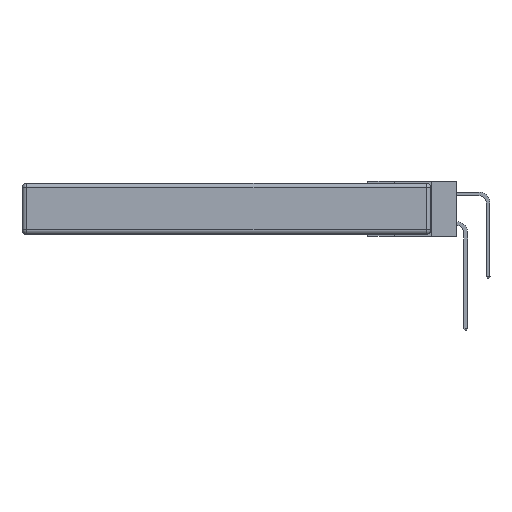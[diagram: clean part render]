
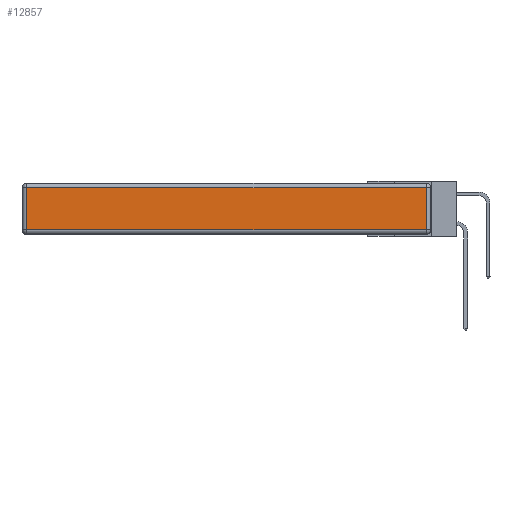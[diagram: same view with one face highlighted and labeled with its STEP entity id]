
A CAD part, left-side view. The second image highlights one B-rep face of the part: STEP entity #12857.
In plain terms, the highlighted planar face has unit normal (-1, 0, 0).
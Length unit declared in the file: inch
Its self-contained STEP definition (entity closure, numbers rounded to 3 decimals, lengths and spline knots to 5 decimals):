
#358 = ORIENTED_EDGE ( 'NONE', *, *, #14253, .T. ) ;
#478 = VERTEX_POINT ( 'NONE', #15212 ) ;
#492 = VECTOR ( 'NONE', #7488, 39.37008 ) ;
#899 = CARTESIAN_POINT ( 'NONE',  ( 0., 2.72, -0.03 ) ) ;
#1174 = ORIENTED_EDGE ( 'NONE', *, *, #6091, .T. ) ;
#2003 = CARTESIAN_POINT ( 'NONE',  ( 0., 2.72, -0.343 ) ) ;
#2862 = CARTESIAN_POINT ( 'NONE',  ( 0., 0., -0.343 ) ) ;
#3069 = LINE ( 'NONE', #8917, #14496 ) ;
#5934 = PLANE ( 'NONE',  #8176 ) ;
#6001 = DIRECTION ( 'NONE',  ( 0., 0., 1. ) ) ;
#6066 = CARTESIAN_POINT ( 'NONE',  ( 0., 0.03, -0.313 ) ) ;
#6091 = EDGE_CURVE ( 'NONE', #9758, #14460, #17847, .T. ) ;
#6378 = VECTOR ( 'NONE', #18759, 39.37008 ) ;
#7292 = CARTESIAN_POINT ( 'NONE',  ( 0., 0.03, -0.343 ) ) ;
#7488 = DIRECTION ( 'NONE',  ( 0., 0., -1. ) ) ;
#7559 = DIRECTION ( 'NONE',  ( -1., 0., 0. ) ) ;
#8176 = AXIS2_PLACEMENT_3D ( 'NONE', #2862, #7559, #6001 ) ;
#8917 = CARTESIAN_POINT ( 'NONE',  ( 0., 2.75, -0.03 ) ) ;
#9630 = LINE ( 'NONE', #7292, #6378 ) ;
#9758 = VERTEX_POINT ( 'NONE', #899 ) ;
#10126 = VECTOR ( 'NONE', #20322, 39.37008 ) ;
#12857 = ADVANCED_FACE ( 'NONE', ( #18185 ), #5934, .T. ) ;
#12870 = CARTESIAN_POINT ( 'NONE',  ( 0., 2.72, -0.313 ) ) ;
#14223 = EDGE_LOOP ( 'NONE', ( #15945, #18724, #358, #1174 ) ) ;
#14253 = EDGE_CURVE ( 'NONE', #478, #9758, #3069, .T. ) ;
#14460 = VERTEX_POINT ( 'NONE', #12870 ) ;
#14496 = VECTOR ( 'NONE', #18626, 39.37008 ) ;
#15029 = LINE ( 'NONE', #17040, #10126 ) ;
#15163 = EDGE_CURVE ( 'NONE', #14460, #15683, #15029, .T. ) ;
#15212 = CARTESIAN_POINT ( 'NONE',  ( 0., 0.03, -0.03 ) ) ;
#15683 = VERTEX_POINT ( 'NONE', #6066 ) ;
#15945 = ORIENTED_EDGE ( 'NONE', *, *, #15163, .T. ) ;
#17040 = CARTESIAN_POINT ( 'NONE',  ( 0., 0., -0.313 ) ) ;
#17847 = LINE ( 'NONE', #2003, #492 ) ;
#18185 = FACE_OUTER_BOUND ( 'NONE', #14223, .T. ) ;
#18626 = DIRECTION ( 'NONE',  ( 0., 1., 0. ) ) ;
#18724 = ORIENTED_EDGE ( 'NONE', *, *, #19939, .T. ) ;
#18759 = DIRECTION ( 'NONE',  ( 0., 0., 1. ) ) ;
#19939 = EDGE_CURVE ( 'NONE', #15683, #478, #9630, .T. ) ;
#20322 = DIRECTION ( 'NONE',  ( 0., -1., 0. ) ) ;
